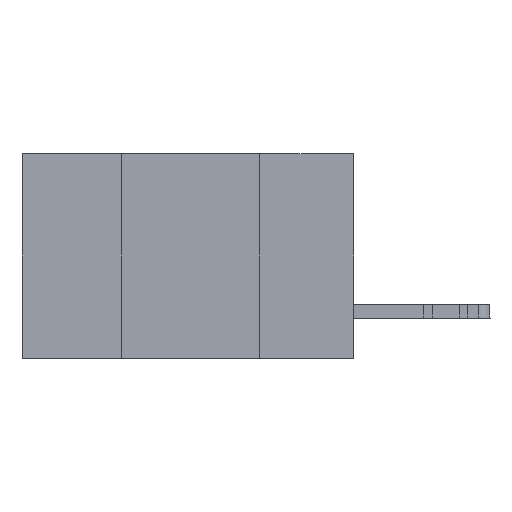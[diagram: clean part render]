
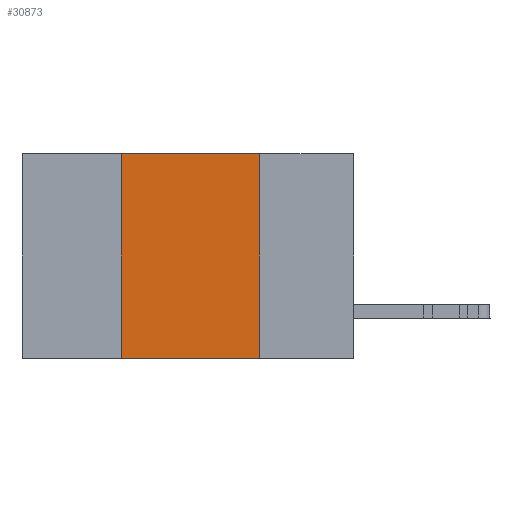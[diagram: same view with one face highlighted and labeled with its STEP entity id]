
A CAD part, left-side view. The second image highlights one B-rep face of the part: STEP entity #30873.
In plain terms, the highlighted planar face has unit normal (-1, 0, 0).
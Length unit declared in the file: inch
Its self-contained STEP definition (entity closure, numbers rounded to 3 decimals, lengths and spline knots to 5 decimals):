
#3142 = AXIS2_PLACEMENT_3D ( 'NONE', #7076, #46722, #42190 ) ;
#3557 = LINE ( 'NONE', #38528, #33920 ) ;
#4249 = EDGE_CURVE ( 'NONE', #41759, #28988, #44176, .T. ) ;
#5154 = FACE_OUTER_BOUND ( 'NONE', #13241, .T. ) ;
#5313 = VECTOR ( 'NONE', #22573, 39.37008 ) ;
#5419 = CARTESIAN_POINT ( 'NONE',  ( 0., 0.42, 0. ) ) ;
#7076 = CARTESIAN_POINT ( 'NONE',  ( 0., 0.6, 0. ) ) ;
#11864 = CARTESIAN_POINT ( 'NONE',  ( 0., 0.17, 0. ) ) ;
#11998 = DIRECTION ( 'NONE',  ( 0., 0., 1. ) ) ;
#12576 = CARTESIAN_POINT ( 'NONE',  ( 0., 0.42, -0.37 ) ) ;
#13241 = EDGE_LOOP ( 'NONE', ( #20518, #37391, #49808, #48201 ) ) ;
#14324 = PLANE ( 'NONE',  #3142 ) ;
#14539 = CARTESIAN_POINT ( 'NONE',  ( 0., 0.6, -0.37 ) ) ;
#14726 = DIRECTION ( 'NONE',  ( 0., -1., 0. ) ) ;
#17135 = LINE ( 'NONE', #27275, #5313 ) ;
#18627 = DIRECTION ( 'NONE',  ( 0., 0., -1. ) ) ;
#20518 = ORIENTED_EDGE ( 'NONE', *, *, #49832, .F. ) ;
#20937 = VECTOR ( 'NONE', #14726, 39.37008 ) ;
#22509 = VECTOR ( 'NONE', #11998, 39.37008 ) ;
#22573 = DIRECTION ( 'NONE',  ( 0., -1., 0. ) ) ;
#26216 = CARTESIAN_POINT ( 'NONE',  ( 0., 0.17, -0.37 ) ) ;
#26656 = VERTEX_POINT ( 'NONE', #11864 ) ;
#27275 = CARTESIAN_POINT ( 'NONE',  ( 0., 0.6, 0. ) ) ;
#28988 = VERTEX_POINT ( 'NONE', #5419 ) ;
#30873 = ADVANCED_FACE ( 'NONE', ( #5154 ), #14324, .F. ) ;
#33920 = VECTOR ( 'NONE', #18627, 39.37008 ) ;
#34006 = EDGE_CURVE ( 'NONE', #41759, #37606, #36490, .T. ) ;
#36490 = LINE ( 'NONE', #14539, #20937 ) ;
#37391 = ORIENTED_EDGE ( 'NONE', *, *, #49867, .F. ) ;
#37606 = VERTEX_POINT ( 'NONE', #26216 ) ;
#38528 = CARTESIAN_POINT ( 'NONE',  ( 0., 0.17, 0. ) ) ;
#41759 = VERTEX_POINT ( 'NONE', #12576 ) ;
#42190 = DIRECTION ( 'NONE',  ( 0., 0., -1. ) ) ;
#44176 = LINE ( 'NONE', #47826, #22509 ) ;
#46722 = DIRECTION ( 'NONE',  ( 1., 0., 0. ) ) ;
#47826 = CARTESIAN_POINT ( 'NONE',  ( 0., 0.42, 0. ) ) ;
#48201 = ORIENTED_EDGE ( 'NONE', *, *, #34006, .T. ) ;
#49808 = ORIENTED_EDGE ( 'NONE', *, *, #4249, .F. ) ;
#49832 = EDGE_CURVE ( 'NONE', #26656, #37606, #3557, .T. ) ;
#49867 = EDGE_CURVE ( 'NONE', #28988, #26656, #17135, .T. ) ;
